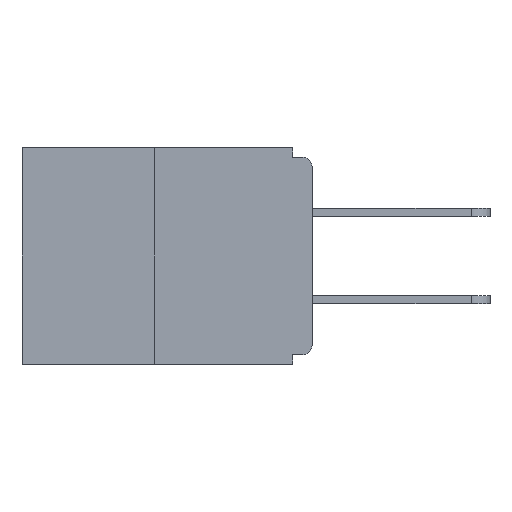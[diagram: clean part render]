
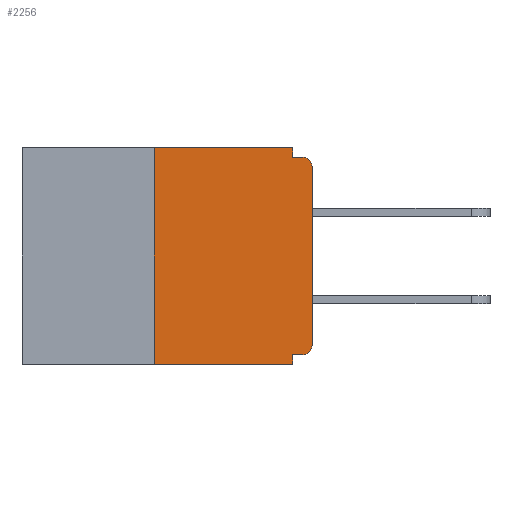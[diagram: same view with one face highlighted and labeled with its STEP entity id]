
A CAD part, left-side view. The second image highlights one B-rep face of the part: STEP entity #2256.
In plain terms, the highlighted planar face has unit normal (-1, 0, 0).
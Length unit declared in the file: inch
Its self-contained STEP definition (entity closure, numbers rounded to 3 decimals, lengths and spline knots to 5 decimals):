
#287 = ORIENTED_EDGE ( 'NONE', *, *, #6977, .F. ) ;
#323 = ORIENTED_EDGE ( 'NONE', *, *, #5693, .T. ) ;
#499 = PLANE ( 'NONE',  #11739 ) ;
#555 = EDGE_CURVE ( 'NONE', #10135, #4135, #2280, .T. ) ;
#557 = VERTEX_POINT ( 'NONE', #8413 ) ;
#594 = CARTESIAN_POINT ( 'NONE',  ( 0., 0.015, -0.313 ) ) ;
#633 = DIRECTION ( 'NONE',  ( -1., 0., 0. ) ) ;
#826 = CARTESIAN_POINT ( 'NONE',  ( 0., 0.031, -0.343 ) ) ;
#834 = CIRCLE ( 'NONE', #7942, 0.015 ) ;
#903 = CIRCLE ( 'NONE', #8626, 0.015 ) ;
#917 = VECTOR ( 'NONE', #9670, 39.37008 ) ;
#918 = LINE ( 'NONE', #6573, #10093 ) ;
#1362 = CARTESIAN_POINT ( 'NONE',  ( 0., 0., -0.03 ) ) ;
#1410 = CARTESIAN_POINT ( 'NONE',  ( 0., 0.46, -0.343 ) ) ;
#1432 = DIRECTION ( 'NONE',  ( 0., 0., 1. ) ) ;
#1535 = DIRECTION ( 'NONE',  ( 0., 0., -1. ) ) ;
#1582 = CARTESIAN_POINT ( 'NONE',  ( 0., 0.46, 0. ) ) ;
#1714 = VERTEX_POINT ( 'NONE', #1362 ) ;
#1842 = CARTESIAN_POINT ( 'NONE',  ( 0., 0.031, -0.343 ) ) ;
#1910 = LINE ( 'NONE', #4468, #9500 ) ;
#1944 = DIRECTION ( 'NONE',  ( 0., 1., 0. ) ) ;
#1964 = CARTESIAN_POINT ( 'NONE',  ( 0., 0., -0.313 ) ) ;
#2214 = EDGE_CURVE ( 'NONE', #4253, #1714, #5396, .T. ) ;
#2224 = DIRECTION ( 'NONE',  ( 0., 0., -1. ) ) ;
#2256 = ADVANCED_FACE ( 'NONE', ( #8511 ), #499, .F. ) ;
#2263 = ORIENTED_EDGE ( 'NONE', *, *, #11622, .F. ) ;
#2280 = LINE ( 'NONE', #1582, #11448 ) ;
#2304 = ORIENTED_EDGE ( 'NONE', *, *, #555, .F. ) ;
#2336 = CARTESIAN_POINT ( 'NONE',  ( 0., 0.25, -0.343 ) ) ;
#2338 = DIRECTION ( 'NONE',  ( 1., 0., 0. ) ) ;
#2507 = EDGE_CURVE ( 'NONE', #2757, #6703, #7870, .T. ) ;
#2634 = DIRECTION ( 'NONE',  ( -1., 0., 0. ) ) ;
#2757 = VERTEX_POINT ( 'NONE', #11225 ) ;
#2795 = VERTEX_POINT ( 'NONE', #9698 ) ;
#2860 = VECTOR ( 'NONE', #1944, 39.37008 ) ;
#3163 = LINE ( 'NONE', #9298, #7739 ) ;
#3705 = EDGE_CURVE ( 'NONE', #2757, #4253, #834, .T. ) ;
#4135 = VERTEX_POINT ( 'NONE', #8035 ) ;
#4203 = VERTEX_POINT ( 'NONE', #1842 ) ;
#4253 = VERTEX_POINT ( 'NONE', #1964 ) ;
#4468 = CARTESIAN_POINT ( 'NONE',  ( 0., 0.25, 0. ) ) ;
#4493 = CARTESIAN_POINT ( 'NONE',  ( 0., 0.015, -0.03 ) ) ;
#4541 = DIRECTION ( 'NONE',  ( 0., 0., 1. ) ) ;
#5396 = LINE ( 'NONE', #10552, #10390 ) ;
#5524 = ORIENTED_EDGE ( 'NONE', *, *, #6021, .F. ) ;
#5561 = DIRECTION ( 'NONE',  ( 0., -1., 0. ) ) ;
#5648 = LINE ( 'NONE', #1410, #10231 ) ;
#5693 = EDGE_CURVE ( 'NONE', #9200, #4203, #5648, .T. ) ;
#5697 = DIRECTION ( 'NONE',  ( 0., -1., 0. ) ) ;
#5733 = EDGE_CURVE ( 'NONE', #6703, #4203, #6777, .T. ) ;
#6021 = EDGE_CURVE ( 'NONE', #9200, #10135, #1910, .T. ) ;
#6573 = CARTESIAN_POINT ( 'NONE',  ( 0., 0.031, 0. ) ) ;
#6615 = DIRECTION ( 'NONE',  ( 0., 0., -1. ) ) ;
#6703 = VERTEX_POINT ( 'NONE', #8782 ) ;
#6777 = LINE ( 'NONE', #826, #917 ) ;
#6932 = ORIENTED_EDGE ( 'NONE', *, *, #3705, .T. ) ;
#6977 = EDGE_CURVE ( 'NONE', #557, #2795, #3163, .T. ) ;
#7461 = EDGE_LOOP ( 'NONE', ( #2304, #5524, #323, #8107, #10003, #6932, #7682, #7479, #287, #2263 ) ) ;
#7479 = ORIENTED_EDGE ( 'NONE', *, *, #11543, .T. ) ;
#7682 = ORIENTED_EDGE ( 'NONE', *, *, #2214, .T. ) ;
#7739 = VECTOR ( 'NONE', #5697, 39.37008 ) ;
#7870 = LINE ( 'NONE', #8214, #2860 ) ;
#7942 = AXIS2_PLACEMENT_3D ( 'NONE', #594, #633, #10696 ) ;
#8035 = CARTESIAN_POINT ( 'NONE',  ( 0., 0.031, 0. ) ) ;
#8107 = ORIENTED_EDGE ( 'NONE', *, *, #5733, .F. ) ;
#8214 = CARTESIAN_POINT ( 'NONE',  ( 0., 0., -0.328 ) ) ;
#8413 = CARTESIAN_POINT ( 'NONE',  ( 0., 0.031, -0.015 ) ) ;
#8511 = FACE_OUTER_BOUND ( 'NONE', #7461, .T. ) ;
#8606 = CARTESIAN_POINT ( 'NONE',  ( 0., 0.46, 0. ) ) ;
#8626 = AXIS2_PLACEMENT_3D ( 'NONE', #4493, #2634, #1535 ) ;
#8782 = CARTESIAN_POINT ( 'NONE',  ( 0., 0.031, -0.328 ) ) ;
#9130 = CARTESIAN_POINT ( 'NONE',  ( 0., 0.25, 0. ) ) ;
#9200 = VERTEX_POINT ( 'NONE', #2336 ) ;
#9298 = CARTESIAN_POINT ( 'NONE',  ( 0., 0., -0.015 ) ) ;
#9500 = VECTOR ( 'NONE', #4541, 39.37008 ) ;
#9670 = DIRECTION ( 'NONE',  ( 0., 0., -1. ) ) ;
#9698 = CARTESIAN_POINT ( 'NONE',  ( 0., 0.015, -0.015 ) ) ;
#10003 = ORIENTED_EDGE ( 'NONE', *, *, #2507, .F. ) ;
#10093 = VECTOR ( 'NONE', #6615, 39.37008 ) ;
#10135 = VERTEX_POINT ( 'NONE', #9130 ) ;
#10231 = VECTOR ( 'NONE', #10394, 39.37008 ) ;
#10390 = VECTOR ( 'NONE', #1432, 39.37008 ) ;
#10394 = DIRECTION ( 'NONE',  ( 0., -1., 0. ) ) ;
#10552 = CARTESIAN_POINT ( 'NONE',  ( 0., 0., 0. ) ) ;
#10696 = DIRECTION ( 'NONE',  ( 0., 0., -1. ) ) ;
#11225 = CARTESIAN_POINT ( 'NONE',  ( 0., 0.015, -0.328 ) ) ;
#11448 = VECTOR ( 'NONE', #5561, 39.37008 ) ;
#11543 = EDGE_CURVE ( 'NONE', #1714, #2795, #903, .T. ) ;
#11622 = EDGE_CURVE ( 'NONE', #4135, #557, #918, .T. ) ;
#11739 = AXIS2_PLACEMENT_3D ( 'NONE', #8606, #2338, #2224 ) ;
